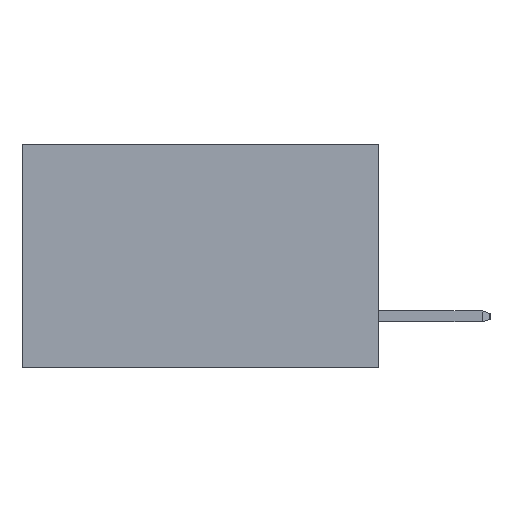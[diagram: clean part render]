
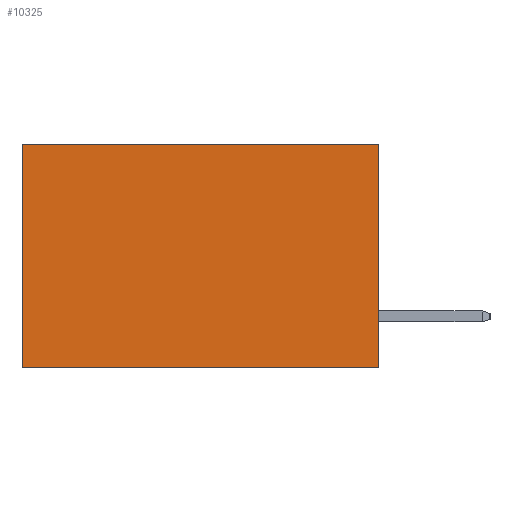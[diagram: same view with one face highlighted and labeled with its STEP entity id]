
A CAD part, left-side view. The second image highlights one B-rep face of the part: STEP entity #10325.
In plain terms, the highlighted planar face has unit normal (-1, 0, 0).
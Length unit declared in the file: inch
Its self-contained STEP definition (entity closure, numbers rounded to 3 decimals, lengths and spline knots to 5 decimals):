
#1468 = VECTOR ( 'NONE', #8842, 39.37008 ) ;
#1573 = DIRECTION ( 'NONE',  ( 0., 0., -1. ) ) ;
#1663 = DIRECTION ( 'NONE',  ( 1., 0., 0. ) ) ;
#1742 = PLANE ( 'NONE',  #15747 ) ;
#1766 = ORIENTED_EDGE ( 'NONE', *, *, #11649, .F. ) ;
#1798 = CARTESIAN_POINT ( 'NONE',  ( 0.277, 0., -0.37 ) ) ;
#2612 = DIRECTION ( 'NONE',  ( 0., 0., -1. ) ) ;
#3054 = CARTESIAN_POINT ( 'NONE',  ( 0.277, 0., -0.37 ) ) ;
#4201 = EDGE_CURVE ( 'NONE', #4216, #5603, #10523, .T. ) ;
#4216 = VERTEX_POINT ( 'NONE', #13611 ) ;
#5603 = VERTEX_POINT ( 'NONE', #12087 ) ;
#6029 = CARTESIAN_POINT ( 'NONE',  ( 0.277, 0., 0. ) ) ;
#6831 = LINE ( 'NONE', #15924, #13213 ) ;
#7882 = ORIENTED_EDGE ( 'NONE', *, *, #4201, .T. ) ;
#8195 = EDGE_CURVE ( 'NONE', #13238, #5603, #6831, .T. ) ;
#8710 = ORIENTED_EDGE ( 'NONE', *, *, #14230, .T. ) ;
#8778 = CARTESIAN_POINT ( 'NONE',  ( 0.277, 0., 0. ) ) ;
#8842 = DIRECTION ( 'NONE',  ( 0., 1., 0. ) ) ;
#10129 = VECTOR ( 'NONE', #14972, 39.37008 ) ;
#10325 = ADVANCED_FACE ( 'NONE', ( #14536 ), #1742, .F. ) ;
#10370 = VECTOR ( 'NONE', #2612, 39.37008 ) ;
#10523 = LINE ( 'NONE', #14774, #10129 ) ;
#10973 = EDGE_LOOP ( 'NONE', ( #7882, #11314, #1766, #8710 ) ) ;
#11314 = ORIENTED_EDGE ( 'NONE', *, *, #8195, .F. ) ;
#11412 = LINE ( 'NONE', #8778, #1468 ) ;
#11649 = EDGE_CURVE ( 'NONE', #13667, #13238, #14096, .T. ) ;
#12087 = CARTESIAN_POINT ( 'NONE',  ( 0.277, 0.59, -0.37 ) ) ;
#12402 = CARTESIAN_POINT ( 'NONE',  ( 0.277, 0., -0.37 ) ) ;
#13213 = VECTOR ( 'NONE', #15737, 39.37008 ) ;
#13238 = VERTEX_POINT ( 'NONE', #12402 ) ;
#13611 = CARTESIAN_POINT ( 'NONE',  ( 0.277, 0.59, 0. ) ) ;
#13667 = VERTEX_POINT ( 'NONE', #6029 ) ;
#14096 = LINE ( 'NONE', #3054, #10370 ) ;
#14230 = EDGE_CURVE ( 'NONE', #13667, #4216, #11412, .T. ) ;
#14536 = FACE_OUTER_BOUND ( 'NONE', #10973, .T. ) ;
#14774 = CARTESIAN_POINT ( 'NONE',  ( 0.277, 0.59, -0.37 ) ) ;
#14972 = DIRECTION ( 'NONE',  ( 0., 0., -1. ) ) ;
#15737 = DIRECTION ( 'NONE',  ( 0., 1., 0. ) ) ;
#15747 = AXIS2_PLACEMENT_3D ( 'NONE', #1798, #1663, #1573 ) ;
#15924 = CARTESIAN_POINT ( 'NONE',  ( 0.277, 0., -0.37 ) ) ;
